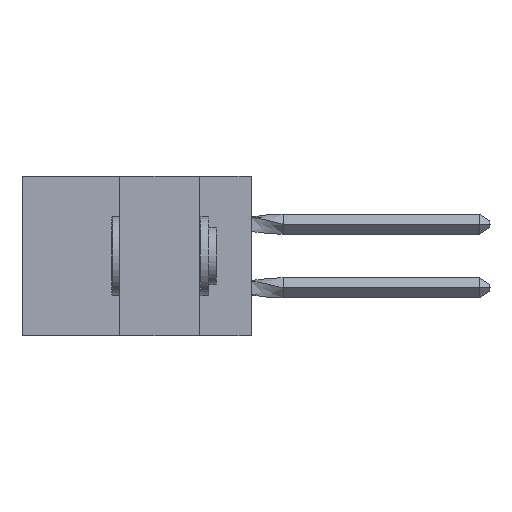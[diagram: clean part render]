
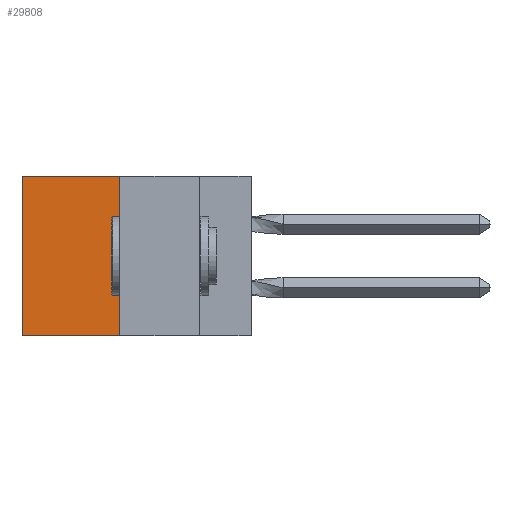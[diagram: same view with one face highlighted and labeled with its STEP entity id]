
A CAD part, left-side view. The second image highlights one B-rep face of the part: STEP entity #29808.
In plain terms, the highlighted planar face has unit normal (-1, 0, 0).
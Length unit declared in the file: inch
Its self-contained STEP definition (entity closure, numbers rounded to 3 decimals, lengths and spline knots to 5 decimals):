
#3495 = LINE ( 'NONE', #10345, #14555 ) ;
#3530 = AXIS2_PLACEMENT_3D ( 'NONE', #24401, #9849, #12281 ) ;
#5334 = DIRECTION ( 'NONE',  ( 0., 1., 0. ) ) ;
#5373 = LINE ( 'NONE', #29685, #23638 ) ;
#7784 = CARTESIAN_POINT ( 'NONE',  ( 0.305, 0.72, 0. ) ) ;
#8362 = ORIENTED_EDGE ( 'NONE', *, *, #12546, .T. ) ;
#9849 = DIRECTION ( 'NONE',  ( 1., 0., 0. ) ) ;
#10345 = CARTESIAN_POINT ( 'NONE',  ( 0.305, 0.413, 0. ) ) ;
#11727 = DIRECTION ( 'NONE',  ( 0., 1., 0. ) ) ;
#11970 = VERTEX_POINT ( 'NONE', #23422 ) ;
#12281 = DIRECTION ( 'NONE',  ( 0., 0., -1. ) ) ;
#12546 = EDGE_CURVE ( 'NONE', #18324, #14253, #3495, .T. ) ;
#12667 = CARTESIAN_POINT ( 'NONE',  ( 0.305, 0.72, -0.5 ) ) ;
#12757 = CARTESIAN_POINT ( 'NONE',  ( 0.305, 0.72, -0.5 ) ) ;
#13890 = ORIENTED_EDGE ( 'NONE', *, *, #14230, .T. ) ;
#14197 = CARTESIAN_POINT ( 'NONE',  ( 0.305, 0.413, 0. ) ) ;
#14230 = EDGE_CURVE ( 'NONE', #14253, #25463, #14877, .T. ) ;
#14253 = VERTEX_POINT ( 'NONE', #7784 ) ;
#14555 = VECTOR ( 'NONE', #5334, 39.37008 ) ;
#14877 = LINE ( 'NONE', #12667, #16388 ) ;
#16388 = VECTOR ( 'NONE', #29754, 39.37008 ) ;
#17481 = EDGE_CURVE ( 'NONE', #18324, #11970, #5373, .T. ) ;
#18324 = VERTEX_POINT ( 'NONE', #14197 ) ;
#18991 = VECTOR ( 'NONE', #11727, 39.37008 ) ;
#19695 = EDGE_LOOP ( 'NONE', ( #13890, #20996, #31235, #8362 ) ) ;
#20996 = ORIENTED_EDGE ( 'NONE', *, *, #29586, .F. ) ;
#21964 = PLANE ( 'NONE',  #3530 ) ;
#22069 = FACE_OUTER_BOUND ( 'NONE', #19695, .T. ) ;
#23422 = CARTESIAN_POINT ( 'NONE',  ( 0.305, 0.413, -0.5 ) ) ;
#23638 = VECTOR ( 'NONE', #30226, 39.37008 ) ;
#24401 = CARTESIAN_POINT ( 'NONE',  ( 0.305, 0.413, -0.5 ) ) ;
#25463 = VERTEX_POINT ( 'NONE', #12757 ) ;
#25480 = LINE ( 'NONE', #26319, #18991 ) ;
#26319 = CARTESIAN_POINT ( 'NONE',  ( 0.305, 0.413, -0.5 ) ) ;
#29586 = EDGE_CURVE ( 'NONE', #11970, #25463, #25480, .T. ) ;
#29685 = CARTESIAN_POINT ( 'NONE',  ( 0.305, 0.413, -0.5 ) ) ;
#29754 = DIRECTION ( 'NONE',  ( 0., 0., -1. ) ) ;
#29808 = ADVANCED_FACE ( 'NONE', ( #22069 ), #21964, .F. ) ;
#30226 = DIRECTION ( 'NONE',  ( 0., 0., -1. ) ) ;
#31235 = ORIENTED_EDGE ( 'NONE', *, *, #17481, .F. ) ;
